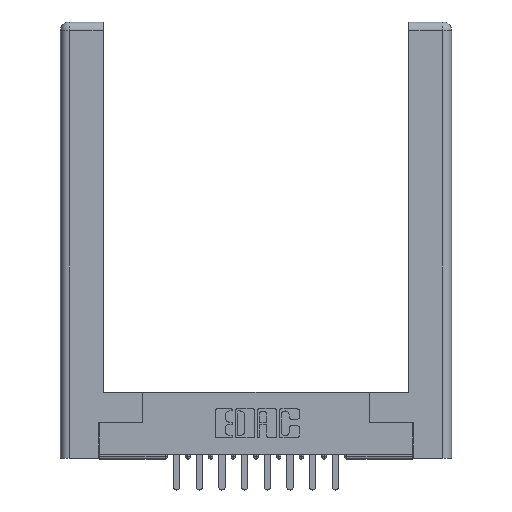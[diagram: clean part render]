
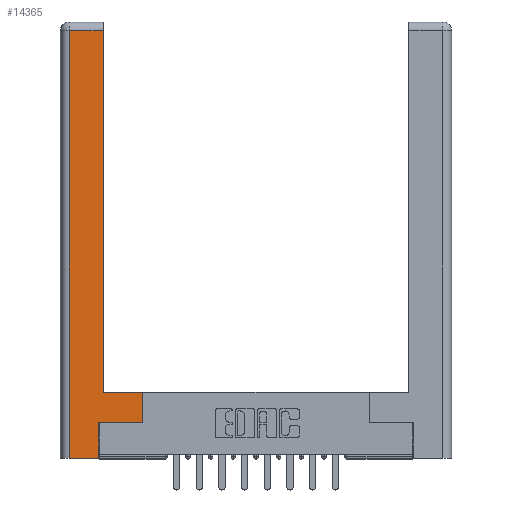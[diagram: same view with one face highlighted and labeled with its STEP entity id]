
A CAD part, top view. The second image highlights one B-rep face of the part: STEP entity #14365.
In plain terms, the highlighted planar face has unit normal (0, 0, 1).
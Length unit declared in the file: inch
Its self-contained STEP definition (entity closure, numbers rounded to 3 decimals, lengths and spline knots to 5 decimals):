
#103 = EDGE_CURVE ( 'NONE', #12081, #870, #8676, .T. ) ;
#130 = DIRECTION ( 'NONE',  ( -1., 0., 0. ) ) ;
#463 = DIRECTION ( 'NONE',  ( -1., 0., 0. ) ) ;
#513 = CARTESIAN_POINT ( 'NONE',  ( 0.295, 0.45, 0. ) ) ;
#526 = VECTOR ( 'NONE', #10915, 39.37008 ) ;
#870 = VERTEX_POINT ( 'NONE', #13546 ) ;
#1021 = CARTESIAN_POINT ( 'NONE',  ( 0.295, 3., 0. ) ) ;
#1092 = DIRECTION ( 'NONE',  ( 0., -1., 0. ) ) ;
#1178 = CARTESIAN_POINT ( 'NONE',  ( 0.295, 0.45, 0. ) ) ;
#1239 = VECTOR ( 'NONE', #463, 39.37008 ) ;
#1254 = DIRECTION ( 'NONE',  ( 0., 0., -1. ) ) ;
#1374 = CARTESIAN_POINT ( 'NONE',  ( 0.295, 2.94, 0. ) ) ;
#1984 = ORIENTED_EDGE ( 'NONE', *, *, #4362, .T. ) ;
#2168 = LINE ( 'NONE', #513, #1239 ) ;
#2241 = VERTEX_POINT ( 'NONE', #6168 ) ;
#2293 = CARTESIAN_POINT ( 'NONE',  ( 0.0615, 0., 0. ) ) ;
#2575 = EDGE_CURVE ( 'NONE', #2241, #3500, #8603, .T. ) ;
#3228 = EDGE_CURVE ( 'NONE', #12870, #2241, #6001, .T. ) ;
#3471 = CARTESIAN_POINT ( 'NONE',  ( 0.265, 0.245, 0. ) ) ;
#3500 = VERTEX_POINT ( 'NONE', #9672 ) ;
#4110 = DIRECTION ( 'NONE',  ( -1., 0., 0. ) ) ;
#4299 = DIRECTION ( 'NONE',  ( 1., 0., 0. ) ) ;
#4362 = EDGE_CURVE ( 'NONE', #5187, #12870, #11147, .T. ) ;
#4741 = VERTEX_POINT ( 'NONE', #1178 ) ;
#4983 = VECTOR ( 'NONE', #12932, 39.37008 ) ;
#5146 = VECTOR ( 'NONE', #5916, 39.37008 ) ;
#5187 = VERTEX_POINT ( 'NONE', #1374 ) ;
#5815 = ORIENTED_EDGE ( 'NONE', *, *, #3228, .T. ) ;
#5916 = DIRECTION ( 'NONE',  ( 0., 1., 0. ) ) ;
#5973 = CARTESIAN_POINT ( 'NONE',  ( 0.265, 0.245, 0. ) ) ;
#6001 = LINE ( 'NONE', #2293, #8036 ) ;
#6042 = PLANE ( 'NONE',  #8290 ) ;
#6103 = EDGE_CURVE ( 'NONE', #4741, #5187, #8296, .T. ) ;
#6168 = CARTESIAN_POINT ( 'NONE',  ( 0.0615, 0., 0. ) ) ;
#6521 = ORIENTED_EDGE ( 'NONE', *, *, #103, .T. ) ;
#7229 = CARTESIAN_POINT ( 'NONE',  ( 0., 0., 0. ) ) ;
#7231 = ORIENTED_EDGE ( 'NONE', *, *, #11406, .T. ) ;
#7365 = EDGE_CURVE ( 'NONE', #3500, #12081, #12564, .T. ) ;
#7449 = CARTESIAN_POINT ( 'NONE',  ( 0.565, 0.45, 0. ) ) ;
#7588 = CARTESIAN_POINT ( 'NONE',  ( 0.0615, 2.94, 0. ) ) ;
#7834 = VERTEX_POINT ( 'NONE', #7449 ) ;
#8036 = VECTOR ( 'NONE', #1092, 39.37008 ) ;
#8290 = AXIS2_PLACEMENT_3D ( 'NONE', #7229, #1254, #130 ) ;
#8296 = LINE ( 'NONE', #1021, #14211 ) ;
#8603 = LINE ( 'NONE', #12798, #10276 ) ;
#8676 = LINE ( 'NONE', #9386, #4983 ) ;
#8758 = CARTESIAN_POINT ( 'NONE',  ( 0.0615, 2.94, 0. ) ) ;
#9102 = DIRECTION ( 'NONE',  ( 0., 1., 0. ) ) ;
#9386 = CARTESIAN_POINT ( 'NONE',  ( 0.565, 0.245, 0. ) ) ;
#9672 = CARTESIAN_POINT ( 'NONE',  ( 0.265, 0., 0. ) ) ;
#9969 = LINE ( 'NONE', #12109, #526 ) ;
#10062 = EDGE_LOOP ( 'NONE', ( #12300, #1984, #5815, #11260, #13662, #6521, #12481, #7231 ) ) ;
#10276 = VECTOR ( 'NONE', #4299, 39.37008 ) ;
#10604 = EDGE_CURVE ( 'NONE', #870, #7834, #9969, .T. ) ;
#10915 = DIRECTION ( 'NONE',  ( 0., 1., 0. ) ) ;
#11147 = LINE ( 'NONE', #8758, #15207 ) ;
#11260 = ORIENTED_EDGE ( 'NONE', *, *, #2575, .T. ) ;
#11406 = EDGE_CURVE ( 'NONE', #7834, #4741, #2168, .T. ) ;
#12081 = VERTEX_POINT ( 'NONE', #3471 ) ;
#12109 = CARTESIAN_POINT ( 'NONE',  ( 0.565, 0.45, 0. ) ) ;
#12300 = ORIENTED_EDGE ( 'NONE', *, *, #6103, .T. ) ;
#12481 = ORIENTED_EDGE ( 'NONE', *, *, #10604, .T. ) ;
#12564 = LINE ( 'NONE', #5973, #5146 ) ;
#12798 = CARTESIAN_POINT ( 'NONE',  ( 0.265, 0., 0. ) ) ;
#12870 = VERTEX_POINT ( 'NONE', #7588 ) ;
#12932 = DIRECTION ( 'NONE',  ( 1., 0., 0. ) ) ;
#13244 = FACE_OUTER_BOUND ( 'NONE', #10062, .T. ) ;
#13546 = CARTESIAN_POINT ( 'NONE',  ( 0.565, 0.245, 0. ) ) ;
#13662 = ORIENTED_EDGE ( 'NONE', *, *, #7365, .T. ) ;
#14211 = VECTOR ( 'NONE', #9102, 39.37008 ) ;
#14365 = ADVANCED_FACE ( 'NONE', ( #13244 ), #6042, .F. ) ;
#15207 = VECTOR ( 'NONE', #4110, 39.37008 ) ;
